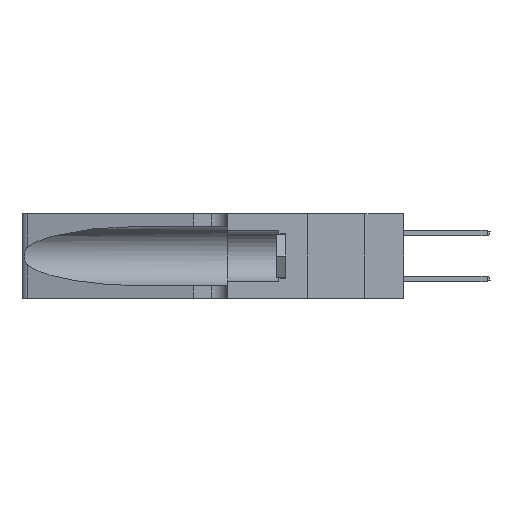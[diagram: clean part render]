
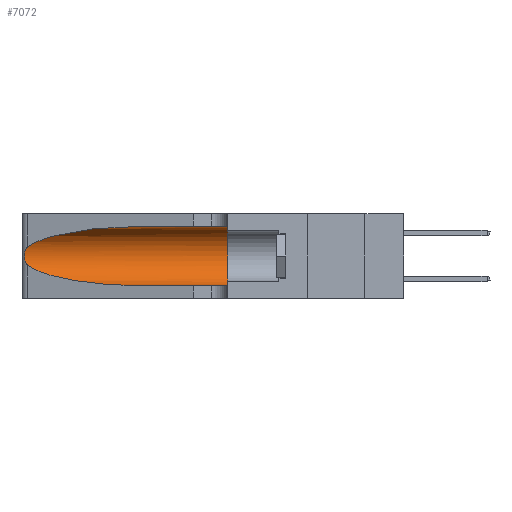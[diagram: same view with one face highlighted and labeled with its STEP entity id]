
A CAD part, left-side view. The second image highlights one B-rep face of the part: STEP entity #7072.
In plain terms, the highlighted cylindrical face has radius 3.308 mm (diameter 6.617 mm), a partial arc.
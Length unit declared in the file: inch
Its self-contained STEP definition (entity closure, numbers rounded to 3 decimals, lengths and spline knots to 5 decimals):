
#280 = CARTESIAN_POINT ( 'NONE',  ( 0.25487, 1.22718, 0.22369 ) ) ;
#412 = EDGE_CURVE ( 'NONE', #25029, #26338, #9750, .T. ) ;
#1416 = CARTESIAN_POINT ( 'NONE',  ( 0.1305, 1.61858, 0.31525 ) ) ;
#1526 = VERTEX_POINT ( 'NONE', #26961 ) ;
#1798 = CARTESIAN_POINT ( 'NONE',  ( 0.1305, 0.72297, 0.31525 ) ) ;
#2077 = CARTESIAN_POINT ( 'NONE',  ( 0.2373, 1.15595, 0.28018 ) ) ;
#2262 = CARTESIAN_POINT ( 'NONE',  ( 0.25487, 1.22718, 0.14631 ) ) ;
#2621 = CARTESIAN_POINT ( 'NONE',  ( 0.18966, 0.96281, 0.05475 ) ) ;
#2793 = ORIENTED_EDGE ( 'NONE', *, *, #3051, .T. ) ;
#3051 = EDGE_CURVE ( 'NONE', #25029, #5163, #3623, .T. ) ;
#3623 =( BOUNDED_CURVE ( )  B_SPLINE_CURVE ( 3, ( #1798, #16945, #2077, #10823 ),
 .UNSPECIFIED., .F., .T. ) 
 B_SPLINE_CURVE_WITH_KNOTS ( ( 4, 4 ),
 ( 1.5708, 2.84003 ),
 .UNSPECIFIED. ) 
 CURVE ( )  GEOMETRIC_REPRESENTATION_ITEM ( )  RATIONAL_B_SPLINE_CURVE ( ( 1., 0.87, 0.87, 1. ) ) 
 REPRESENTATION_ITEM ( '' )  );
#3920 = AXIS2_PLACEMENT_3D ( 'NONE', #15909, #24505, #15083 ) ;
#4421 = CARTESIAN_POINT ( 'NONE',  ( 0.25555, 1.22994, 0.2215 ) ) ;
#4785 = CYLINDRICAL_SURFACE ( 'NONE', #11105, 0.13025 ) ;
#4856 = CARTESIAN_POINT ( 'NONE',  ( 0.26075, 1.23896, 0.19203 ) ) ;
#5051 = VERTEX_POINT ( 'NONE', #26653 ) ;
#5163 = VERTEX_POINT ( 'NONE', #10492 ) ;
#6731 = LINE ( 'NONE', #7274, #17976 ) ;
#7072 = ADVANCED_FACE ( 'NONE', ( #10606 ), #4785, .F. ) ;
#7274 = CARTESIAN_POINT ( 'NONE',  ( 0.1305, 1.61858, 0.05475 ) ) ;
#7845 = EDGE_LOOP ( 'NONE', ( #2793, #23249, #22405, #15268, #8926, #9033 ) ) ;
#8926 = ORIENTED_EDGE ( 'NONE', *, *, #9383, .F. ) ;
#9033 = ORIENTED_EDGE ( 'NONE', *, *, #412, .F. ) ;
#9286 = DIRECTION ( 'NONE',  ( 0., 0., -1. ) ) ;
#9287 = CARTESIAN_POINT ( 'NONE',  ( 0.2373, 1.15595, 0.08982 ) ) ;
#9383 = EDGE_CURVE ( 'NONE', #26338, #5051, #21060, .T. ) ;
#9417 = CARTESIAN_POINT ( 'NONE',  ( 0.25639, 1.23184, 0.21858 ) ) ;
#9481 = DIRECTION ( 'NONE',  ( 0., -1., 0. ) ) ;
#9750 = LINE ( 'NONE', #1416, #21701 ) ;
#9755 = CARTESIAN_POINT ( 'NONE',  ( 0.1305, 0.72297, 0.05475 ) ) ;
#10486 = VERTEX_POINT ( 'NONE', #9755 ) ;
#10492 = CARTESIAN_POINT ( 'NONE',  ( 0.25487, 1.22718, 0.22369 ) ) ;
#10606 = FACE_OUTER_BOUND ( 'NONE', #7845, .T. ) ;
#10823 = CARTESIAN_POINT ( 'NONE',  ( 0.25487, 1.22718, 0.22369 ) ) ;
#11105 = AXIS2_PLACEMENT_3D ( 'NONE', #15968, #9481, #9286 ) ;
#12196 = CARTESIAN_POINT ( 'NONE',  ( 0.1305, 0.35, 0.31525 ) ) ;
#13213 =( BOUNDED_CURVE ( )  B_SPLINE_CURVE ( 3, ( #2262, #9287, #2621, #20342 ),
 .UNSPECIFIED., .F., .F. ) 
 B_SPLINE_CURVE_WITH_KNOTS ( ( 4, 4 ),
 ( 3.44316, 4.71239 ),
 .UNSPECIFIED. ) 
 CURVE ( )  GEOMETRIC_REPRESENTATION_ITEM ( )  RATIONAL_B_SPLINE_CURVE ( ( 1., 0.87, 0.87, 1. ) ) 
 REPRESENTATION_ITEM ( '' )  );
#14467 = CARTESIAN_POINT ( 'NONE',  ( 0.25639, 1.23186, 0.15144 ) ) ;
#14480 = EDGE_CURVE ( 'NONE', #1526, #10486, #13213, .T. ) ;
#14660 = CARTESIAN_POINT ( 'NONE',  ( 0.1305, 0.72297, 0.31525 ) ) ;
#15083 = DIRECTION ( 'NONE',  ( 0., 0., 1. ) ) ;
#15268 = ORIENTED_EDGE ( 'NONE', *, *, #21859, .T. ) ;
#15719 = CARTESIAN_POINT ( 'NONE',  ( 0.26075, 1.23896, 0.178 ) ) ;
#15909 = CARTESIAN_POINT ( 'NONE',  ( 0.1305, 0.35, 0.185 ) ) ;
#15968 = CARTESIAN_POINT ( 'NONE',  ( 0.1305, 1.61858, 0.185 ) ) ;
#16657 = DIRECTION ( 'NONE',  ( 0., -1., 0. ) ) ;
#16945 = CARTESIAN_POINT ( 'NONE',  ( 0.18966, 0.96281, 0.31525 ) ) ;
#17080 = B_SPLINE_CURVE_WITH_KNOTS ( 'NONE', 3,
 ( #280, #4421, #9417, #24602, #17806, #24320, #4856, #15719, #25160, #21224, #18931, #14467, #27362, #18746 ),
 .UNSPECIFIED., .F., .F.,
 ( 4, 2, 2, 2, 2, 2, 4 ),
 ( 0., 0.00027, 0.00053, 0.00107, 0.0016, 0.00187, 0.00214 ),
 .UNSPECIFIED. ) ;
#17806 = CARTESIAN_POINT ( 'NONE',  ( 0.25854, 1.2359, 0.20912 ) ) ;
#17976 = VECTOR ( 'NONE', #18824, 39.37008 ) ;
#18746 = CARTESIAN_POINT ( 'NONE',  ( 0.25487, 1.22718, 0.14631 ) ) ;
#18824 = DIRECTION ( 'NONE',  ( 0., -1., 0. ) ) ;
#18931 = CARTESIAN_POINT ( 'NONE',  ( 0.25789, 1.23486, 0.15765 ) ) ;
#20342 = CARTESIAN_POINT ( 'NONE',  ( 0.1305, 0.72297, 0.05475 ) ) ;
#21060 = CIRCLE ( 'NONE', #3920, 0.13025 ) ;
#21224 = CARTESIAN_POINT ( 'NONE',  ( 0.25856, 1.23593, 0.16098 ) ) ;
#21701 = VECTOR ( 'NONE', #16657, 39.37008 ) ;
#21859 = EDGE_CURVE ( 'NONE', #10486, #5051, #6731, .T. ) ;
#22405 = ORIENTED_EDGE ( 'NONE', *, *, #14480, .T. ) ;
#23113 = EDGE_CURVE ( 'NONE', #5163, #1526, #17080, .T. ) ;
#23249 = ORIENTED_EDGE ( 'NONE', *, *, #23113, .T. ) ;
#24320 = CARTESIAN_POINT ( 'NONE',  ( 0.26018, 1.23835, 0.19895 ) ) ;
#24505 = DIRECTION ( 'NONE',  ( 0., 1., 0. ) ) ;
#24602 = CARTESIAN_POINT ( 'NONE',  ( 0.25787, 1.23484, 0.2124 ) ) ;
#25029 = VERTEX_POINT ( 'NONE', #14660 ) ;
#25160 = CARTESIAN_POINT ( 'NONE',  ( 0.26017, 1.23833, 0.17102 ) ) ;
#26338 = VERTEX_POINT ( 'NONE', #12196 ) ;
#26653 = CARTESIAN_POINT ( 'NONE',  ( 0.1305, 0.35, 0.05475 ) ) ;
#26961 = CARTESIAN_POINT ( 'NONE',  ( 0.25487, 1.22718, 0.14631 ) ) ;
#27362 = CARTESIAN_POINT ( 'NONE',  ( 0.25555, 1.22993, 0.14849 ) ) ;
